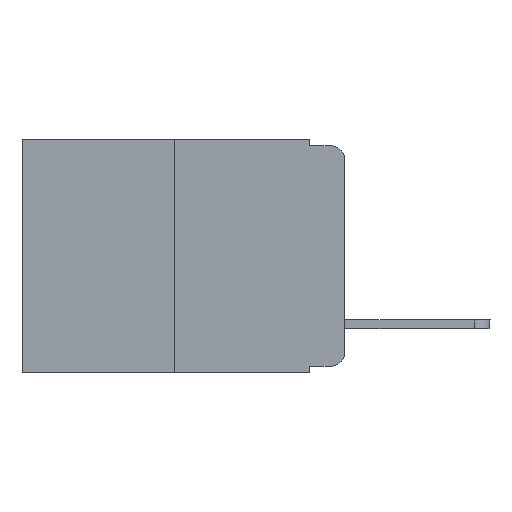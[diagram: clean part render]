
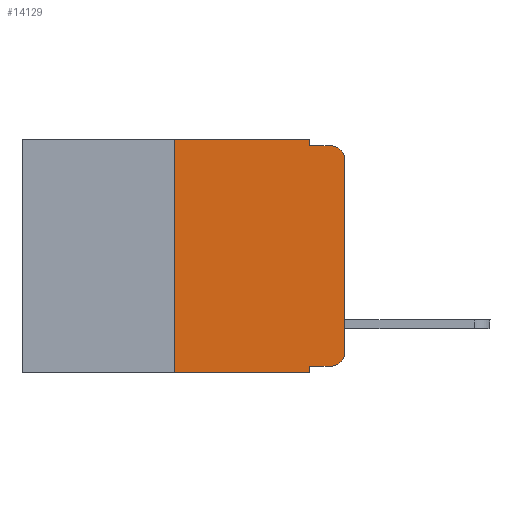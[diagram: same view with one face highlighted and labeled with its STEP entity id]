
A CAD part, left-side view. The second image highlights one B-rep face of the part: STEP entity #14129.
In plain terms, the highlighted planar face has unit normal (-1, 0, 0).
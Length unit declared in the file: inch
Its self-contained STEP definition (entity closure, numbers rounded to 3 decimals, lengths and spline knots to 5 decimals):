
#159 = VERTEX_POINT ( 'NONE', #1164 ) ;
#412 = PLANE ( 'NONE',  #13152 ) ;
#1164 = CARTESIAN_POINT ( 'NONE',  ( 0., 0.051, 0. ) ) ;
#1500 = EDGE_CURVE ( 'NONE', #8006, #3507, #4478, .T. ) ;
#1894 = CARTESIAN_POINT ( 'NONE',  ( 0., 0.051, -0.343 ) ) ;
#1898 = FACE_OUTER_BOUND ( 'NONE', #5677, .T. ) ;
#1908 = LINE ( 'NONE', #3479, #5202 ) ;
#1914 = DIRECTION ( 'NONE',  ( -1., 0., 0. ) ) ;
#2027 = EDGE_CURVE ( 'NONE', #17642, #13542, #13335, .T. ) ;
#2320 = EDGE_CURVE ( 'NONE', #10029, #6013, #18676, .T. ) ;
#2343 = CARTESIAN_POINT ( 'NONE',  ( 0., 0.051, -0.333 ) ) ;
#2784 = VERTEX_POINT ( 'NONE', #2343 ) ;
#3129 = EDGE_CURVE ( 'NONE', #3507, #10029, #13546, .T. ) ;
#3382 = ORIENTED_EDGE ( 'NONE', *, *, #13055, .F. ) ;
#3399 = CARTESIAN_POINT ( 'NONE',  ( 0., 0., -0.03 ) ) ;
#3479 = CARTESIAN_POINT ( 'NONE',  ( 0., 0.051, -0.01 ) ) ;
#3507 = VERTEX_POINT ( 'NONE', #9190 ) ;
#3737 = CARTESIAN_POINT ( 'NONE',  ( 0., 0.473, 0. ) ) ;
#4470 = LINE ( 'NONE', #16408, #7511 ) ;
#4478 = CIRCLE ( 'NONE', #13536, 0.02 ) ;
#5202 = VECTOR ( 'NONE', #20045, 39.37008 ) ;
#5415 = LINE ( 'NONE', #15297, #17876 ) ;
#5570 = DIRECTION ( 'NONE',  ( 0., -1., 0. ) ) ;
#5677 = EDGE_LOOP ( 'NONE', ( #15336, #6245, #6984, #18386, #10730, #19827, #11241, #3382, #13527, #6053 ) ) ;
#5740 = DIRECTION ( 'NONE',  ( 0., 0., 1. ) ) ;
#6013 = VERTEX_POINT ( 'NONE', #9925 ) ;
#6053 = ORIENTED_EDGE ( 'NONE', *, *, #1500, .T. ) ;
#6088 = DIRECTION ( 'NONE',  ( 0., -1., 0. ) ) ;
#6245 = ORIENTED_EDGE ( 'NONE', *, *, #2320, .T. ) ;
#6342 = CARTESIAN_POINT ( 'NONE',  ( 0., 0., 0. ) ) ;
#6498 = LINE ( 'NONE', #10745, #16423 ) ;
#6608 = VERTEX_POINT ( 'NONE', #17787 ) ;
#6984 = ORIENTED_EDGE ( 'NONE', *, *, #7474, .F. ) ;
#7039 = EDGE_CURVE ( 'NONE', #13542, #159, #4470, .T. ) ;
#7474 = EDGE_CURVE ( 'NONE', #6608, #6013, #1908, .T. ) ;
#7511 = VECTOR ( 'NONE', #11650, 39.37008 ) ;
#8006 = VERTEX_POINT ( 'NONE', #8715 ) ;
#8105 = CARTESIAN_POINT ( 'NONE',  ( 0., 0.25, -0.343 ) ) ;
#8405 = CARTESIAN_POINT ( 'NONE',  ( 0., 0.25, 0. ) ) ;
#8715 = CARTESIAN_POINT ( 'NONE',  ( 0., 0.02, -0.333 ) ) ;
#8993 = EDGE_CURVE ( 'NONE', #2784, #8006, #5415, .T. ) ;
#9190 = CARTESIAN_POINT ( 'NONE',  ( 0., 0., -0.313 ) ) ;
#9675 = DIRECTION ( 'NONE',  ( 0., 0., 1. ) ) ;
#9925 = CARTESIAN_POINT ( 'NONE',  ( 0., 0.02, -0.01 ) ) ;
#10029 = VERTEX_POINT ( 'NONE', #3399 ) ;
#10221 = VERTEX_POINT ( 'NONE', #1894 ) ;
#10730 = ORIENTED_EDGE ( 'NONE', *, *, #7039, .F. ) ;
#10745 = CARTESIAN_POINT ( 'NONE',  ( 0., 0.051, 0. ) ) ;
#11241 = ORIENTED_EDGE ( 'NONE', *, *, #13942, .T. ) ;
#11592 = LINE ( 'NONE', #13520, #17193 ) ;
#11650 = DIRECTION ( 'NONE',  ( 0., -1., 0. ) ) ;
#12080 = VECTOR ( 'NONE', #6088, 39.37008 ) ;
#12294 = CARTESIAN_POINT ( 'NONE',  ( 0., 0.25, 0. ) ) ;
#13055 = EDGE_CURVE ( 'NONE', #2784, #10221, #6498, .T. ) ;
#13152 = AXIS2_PLACEMENT_3D ( 'NONE', #3737, #14999, #13584 ) ;
#13335 = LINE ( 'NONE', #12294, #18941 ) ;
#13520 = CARTESIAN_POINT ( 'NONE',  ( 0., 0.051, 0. ) ) ;
#13527 = ORIENTED_EDGE ( 'NONE', *, *, #8993, .T. ) ;
#13536 = AXIS2_PLACEMENT_3D ( 'NONE', #14890, #1914, #16541 ) ;
#13542 = VERTEX_POINT ( 'NONE', #8405 ) ;
#13546 = LINE ( 'NONE', #6342, #20177 ) ;
#13584 = DIRECTION ( 'NONE',  ( 0., 0., -1. ) ) ;
#13942 = EDGE_CURVE ( 'NONE', #17642, #10221, #17429, .T. ) ;
#14072 = DIRECTION ( 'NONE',  ( 0., 0., -1. ) ) ;
#14129 = ADVANCED_FACE ( 'NONE', ( #1898 ), #412, .F. ) ;
#14556 = EDGE_CURVE ( 'NONE', #159, #6608, #11592, .T. ) ;
#14890 = CARTESIAN_POINT ( 'NONE',  ( 0., 0.02, -0.313 ) ) ;
#14925 = DIRECTION ( 'NONE',  ( 0., 0., -1. ) ) ;
#14999 = DIRECTION ( 'NONE',  ( 1., 0., 0. ) ) ;
#15297 = CARTESIAN_POINT ( 'NONE',  ( 0., 0.051, -0.333 ) ) ;
#15336 = ORIENTED_EDGE ( 'NONE', *, *, #3129, .T. ) ;
#15824 = DIRECTION ( 'NONE',  ( -1., 0., 0. ) ) ;
#16408 = CARTESIAN_POINT ( 'NONE',  ( 0., 0.473, 0. ) ) ;
#16423 = VECTOR ( 'NONE', #20364, 39.37008 ) ;
#16541 = DIRECTION ( 'NONE',  ( 0., 0., -1. ) ) ;
#17193 = VECTOR ( 'NONE', #14925, 39.37008 ) ;
#17275 = CARTESIAN_POINT ( 'NONE',  ( 0., 0.473, -0.343 ) ) ;
#17429 = LINE ( 'NONE', #17275, #12080 ) ;
#17642 = VERTEX_POINT ( 'NONE', #8105 ) ;
#17787 = CARTESIAN_POINT ( 'NONE',  ( 0., 0.051, -0.01 ) ) ;
#17876 = VECTOR ( 'NONE', #5570, 39.37008 ) ;
#18386 = ORIENTED_EDGE ( 'NONE', *, *, #14556, .F. ) ;
#18676 = CIRCLE ( 'NONE', #21021, 0.02 ) ;
#18941 = VECTOR ( 'NONE', #5740, 39.37008 ) ;
#19049 = CARTESIAN_POINT ( 'NONE',  ( 0., 0.02, -0.03 ) ) ;
#19827 = ORIENTED_EDGE ( 'NONE', *, *, #2027, .F. ) ;
#20045 = DIRECTION ( 'NONE',  ( 0., -1., 0. ) ) ;
#20177 = VECTOR ( 'NONE', #9675, 39.37008 ) ;
#20364 = DIRECTION ( 'NONE',  ( 0., 0., -1. ) ) ;
#21021 = AXIS2_PLACEMENT_3D ( 'NONE', #19049, #15824, #14072 ) ;
